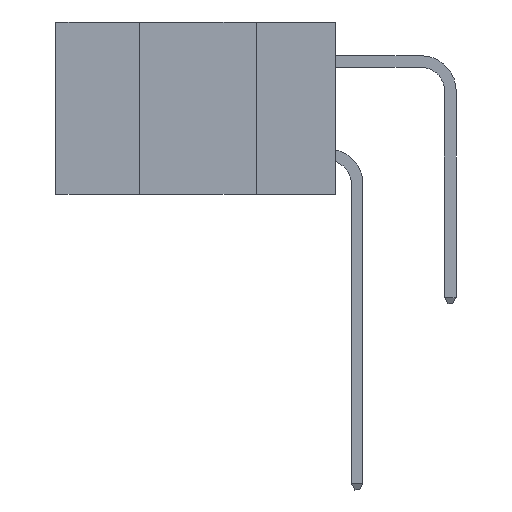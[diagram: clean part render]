
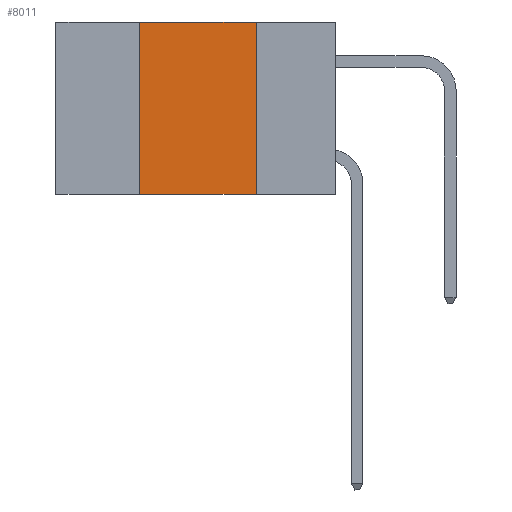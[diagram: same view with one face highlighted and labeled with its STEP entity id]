
A CAD part, left-side view. The second image highlights one B-rep face of the part: STEP entity #8011.
In plain terms, the highlighted planar face has unit normal (-1, 0, 0).
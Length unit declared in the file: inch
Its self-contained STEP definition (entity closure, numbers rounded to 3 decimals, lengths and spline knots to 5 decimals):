
#320 = CARTESIAN_POINT ( 'NONE',  ( 0., 0.6, 0. ) ) ;
#382 = DIRECTION ( 'NONE',  ( 0., 0., -1. ) ) ;
#384 = ORIENTED_EDGE ( 'NONE', *, *, #9969, .F. ) ;
#651 = ORIENTED_EDGE ( 'NONE', *, *, #3006, .F. ) ;
#983 = VERTEX_POINT ( 'NONE', #5071 ) ;
#1116 = EDGE_LOOP ( 'NONE', ( #8864, #651, #384, #6063 ) ) ;
#2210 = DIRECTION ( 'NONE',  ( 1., 0., 0. ) ) ;
#2319 = DIRECTION ( 'NONE',  ( 0., -1., 0. ) ) ;
#2358 = EDGE_CURVE ( 'NONE', #8594, #9554, #2902, .T. ) ;
#2593 = CARTESIAN_POINT ( 'NONE',  ( 0., 0.17, -0.37 ) ) ;
#2735 = VECTOR ( 'NONE', #2319, 39.37008 ) ;
#2902 = LINE ( 'NONE', #7039, #11626 ) ;
#3006 = EDGE_CURVE ( 'NONE', #983, #8594, #5541, .T. ) ;
#3479 = DIRECTION ( 'NONE',  ( 0., 0., 1. ) ) ;
#3534 = LINE ( 'NONE', #3825, #8147 ) ;
#3825 = CARTESIAN_POINT ( 'NONE',  ( 0., 0.6, -0.37 ) ) ;
#4080 = PLANE ( 'NONE',  #8317 ) ;
#4249 = FACE_OUTER_BOUND ( 'NONE', #1116, .T. ) ;
#4758 = DIRECTION ( 'NONE',  ( 0., -1., 0. ) ) ;
#4991 = CARTESIAN_POINT ( 'NONE',  ( 0., 0.42, -0.37 ) ) ;
#5071 = CARTESIAN_POINT ( 'NONE',  ( 0., 0.42, 0. ) ) ;
#5541 = LINE ( 'NONE', #320, #2735 ) ;
#6063 = ORIENTED_EDGE ( 'NONE', *, *, #7814, .T. ) ;
#6520 = VECTOR ( 'NONE', #3479, 39.37008 ) ;
#7039 = CARTESIAN_POINT ( 'NONE',  ( 0., 0.17, 0. ) ) ;
#7814 = EDGE_CURVE ( 'NONE', #11361, #9554, #3534, .T. ) ;
#8011 = ADVANCED_FACE ( 'NONE', ( #4249 ), #4080, .F. ) ;
#8147 = VECTOR ( 'NONE', #4758, 39.37008 ) ;
#8317 = AXIS2_PLACEMENT_3D ( 'NONE', #10389, #2210, #8714 ) ;
#8594 = VERTEX_POINT ( 'NONE', #11165 ) ;
#8714 = DIRECTION ( 'NONE',  ( 0., 0., -1. ) ) ;
#8864 = ORIENTED_EDGE ( 'NONE', *, *, #2358, .F. ) ;
#9554 = VERTEX_POINT ( 'NONE', #2593 ) ;
#9845 = CARTESIAN_POINT ( 'NONE',  ( 0., 0.42, 0. ) ) ;
#9969 = EDGE_CURVE ( 'NONE', #11361, #983, #11440, .T. ) ;
#10389 = CARTESIAN_POINT ( 'NONE',  ( 0., 0.6, 0. ) ) ;
#11165 = CARTESIAN_POINT ( 'NONE',  ( 0., 0.17, 0. ) ) ;
#11361 = VERTEX_POINT ( 'NONE', #4991 ) ;
#11440 = LINE ( 'NONE', #9845, #6520 ) ;
#11626 = VECTOR ( 'NONE', #382, 39.37008 ) ;
